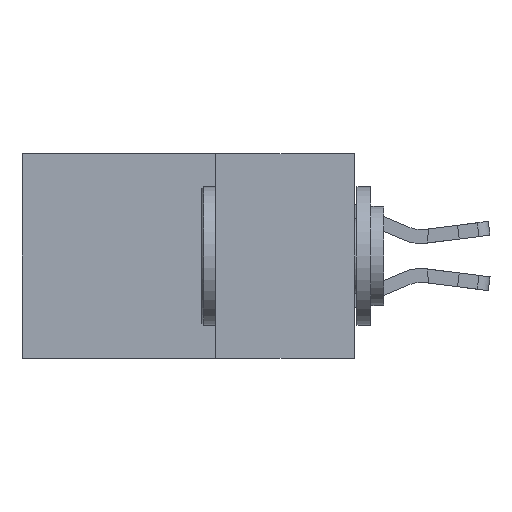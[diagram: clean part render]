
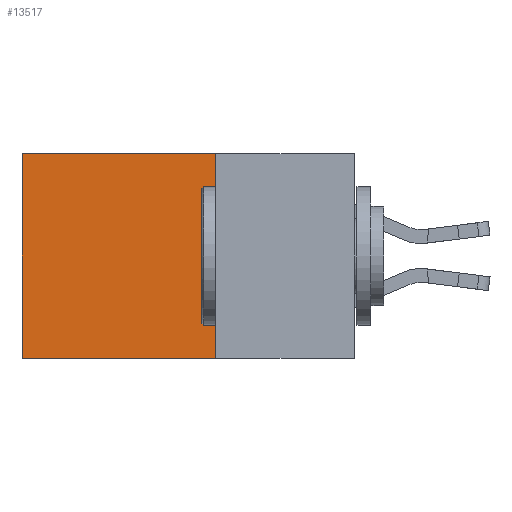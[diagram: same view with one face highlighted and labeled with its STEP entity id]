
A CAD part, left-side view. The second image highlights one B-rep face of the part: STEP entity #13517.
In plain terms, the highlighted planar face has unit normal (-1, 0, 0).
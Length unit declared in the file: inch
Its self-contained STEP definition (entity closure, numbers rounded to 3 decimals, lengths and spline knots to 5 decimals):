
#152 = VECTOR ( 'NONE', #530, 39.37008 ) ;
#417 = CARTESIAN_POINT ( 'NONE',  ( 0.298, 0.25, 0. ) ) ;
#530 = DIRECTION ( 'NONE',  ( 0., 1., 0. ) ) ;
#590 = CARTESIAN_POINT ( 'NONE',  ( 0.298, 0.25, 0. ) ) ;
#1173 = VERTEX_POINT ( 'NONE', #1996 ) ;
#1330 = VERTEX_POINT ( 'NONE', #14014 ) ;
#1849 = CARTESIAN_POINT ( 'NONE',  ( 0.298, 0.25, 0. ) ) ;
#1996 = CARTESIAN_POINT ( 'NONE',  ( 0.298, 0.6, 0. ) ) ;
#2260 = ORIENTED_EDGE ( 'NONE', *, *, #16171, .T. ) ;
#2578 = VERTEX_POINT ( 'NONE', #15330 ) ;
#2594 = ORIENTED_EDGE ( 'NONE', *, *, #16111, .T. ) ;
#3712 = PLANE ( 'NONE',  #7510 ) ;
#3777 = DIRECTION ( 'NONE',  ( 0., 0., -1. ) ) ;
#4885 = ORIENTED_EDGE ( 'NONE', *, *, #14501, .F. ) ;
#4891 = VERTEX_POINT ( 'NONE', #590 ) ;
#5233 = CARTESIAN_POINT ( 'NONE',  ( 0.298, 0.25, -0.37 ) ) ;
#5386 = LINE ( 'NONE', #5639, #12509 ) ;
#5583 = LINE ( 'NONE', #417, #152 ) ;
#5608 = DIRECTION ( 'NONE',  ( 0., 0., -1. ) ) ;
#5639 = CARTESIAN_POINT ( 'NONE',  ( 0.298, 0.6, 0. ) ) ;
#7510 = AXIS2_PLACEMENT_3D ( 'NONE', #11542, #10121, #3777 ) ;
#8419 = VECTOR ( 'NONE', #5608, 39.37008 ) ;
#9238 = EDGE_CURVE ( 'NONE', #4891, #2578, #11883, .T. ) ;
#10121 = DIRECTION ( 'NONE',  ( 1., 0., 0. ) ) ;
#10910 = LINE ( 'NONE', #5233, #14610 ) ;
#11542 = CARTESIAN_POINT ( 'NONE',  ( 0.298, 0.25, 0. ) ) ;
#11883 = LINE ( 'NONE', #1849, #8419 ) ;
#12395 = EDGE_LOOP ( 'NONE', ( #2594, #4885, #15920, #2260 ) ) ;
#12509 = VECTOR ( 'NONE', #16097, 39.37008 ) ;
#13517 = ADVANCED_FACE ( 'NONE', ( #14217 ), #3712, .F. ) ;
#14014 = CARTESIAN_POINT ( 'NONE',  ( 0.298, 0.6, -0.37 ) ) ;
#14217 = FACE_OUTER_BOUND ( 'NONE', #12395, .T. ) ;
#14501 = EDGE_CURVE ( 'NONE', #2578, #1330, #10910, .T. ) ;
#14610 = VECTOR ( 'NONE', #15476, 39.37008 ) ;
#15330 = CARTESIAN_POINT ( 'NONE',  ( 0.298, 0.25, -0.37 ) ) ;
#15476 = DIRECTION ( 'NONE',  ( 0., 1., 0. ) ) ;
#15920 = ORIENTED_EDGE ( 'NONE', *, *, #9238, .F. ) ;
#16097 = DIRECTION ( 'NONE',  ( 0., 0., -1. ) ) ;
#16111 = EDGE_CURVE ( 'NONE', #1173, #1330, #5386, .T. ) ;
#16171 = EDGE_CURVE ( 'NONE', #4891, #1173, #5583, .T. ) ;
